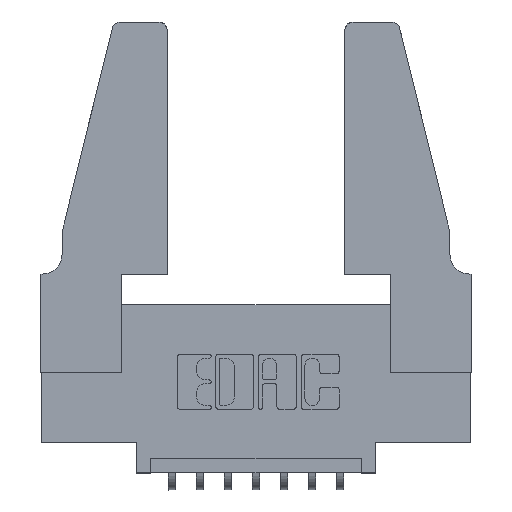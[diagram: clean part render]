
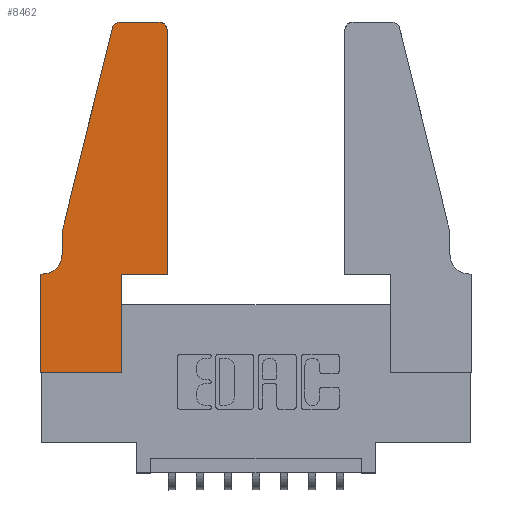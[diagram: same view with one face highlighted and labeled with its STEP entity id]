
A CAD part, top view. The second image highlights one B-rep face of the part: STEP entity #8462.
In plain terms, the highlighted planar face has unit normal (0, 0, 1).
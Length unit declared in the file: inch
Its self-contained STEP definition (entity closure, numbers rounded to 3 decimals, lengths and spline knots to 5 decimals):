
#113 = ORIENTED_EDGE ( 'NONE', *, *, #2184, .T. ) ;
#610 = VERTEX_POINT ( 'NONE', #11148 ) ;
#645 = DIRECTION ( 'NONE',  ( 0., 0., 1. ) ) ;
#992 = DIRECTION ( 'NONE',  ( -0.239, -0.971, 0. ) ) ;
#1128 = VERTEX_POINT ( 'NONE', #3103 ) ;
#1133 = CARTESIAN_POINT ( 'NONE',  ( 0.25487, 1.22718, 0.37 ) ) ;
#1304 = VECTOR ( 'NONE', #4880, 39.37008 ) ;
#1329 = EDGE_CURVE ( 'NONE', #610, #11386, #11660, .T. ) ;
#1362 = VERTEX_POINT ( 'NONE', #4406 ) ;
#1475 = CARTESIAN_POINT ( 'NONE',  ( 0.4505, 0.35, 0.37 ) ) ;
#1483 = VECTOR ( 'NONE', #10228, 39.37008 ) ;
#1531 = DIRECTION ( 'NONE',  ( 1., 0., 0. ) ) ;
#1594 = CARTESIAN_POINT ( 'NONE',  ( 0.0755, 0.5, 0.37 ) ) ;
#1610 = LINE ( 'NONE', #6700, #1304 ) ;
#2184 = EDGE_CURVE ( 'NONE', #7097, #1362, #9536, .T. ) ;
#2194 = ORIENTED_EDGE ( 'NONE', *, *, #4125, .T. ) ;
#2201 = ORIENTED_EDGE ( 'NONE', *, *, #6416, .T. ) ;
#2238 = VECTOR ( 'NONE', #10749, 39.37008 ) ;
#2318 = CARTESIAN_POINT ( 'NONE',  ( 0.4505, 0.35, 0.37 ) ) ;
#2446 = ORIENTED_EDGE ( 'NONE', *, *, #8698, .T. ) ;
#2585 = CARTESIAN_POINT ( 'NONE',  ( 0., 0., 0.37 ) ) ;
#2782 = CARTESIAN_POINT ( 'NONE',  ( 0.4505, 1.22, 0.37 ) ) ;
#3103 = CARTESIAN_POINT ( 'NONE',  ( 0.2865, 0.35, 0.37 ) ) ;
#3108 = CARTESIAN_POINT ( 'NONE',  ( 0.0755, 0.5, 0.37 ) ) ;
#3362 = DIRECTION ( 'NONE',  ( 0., 0., 1. ) ) ;
#3425 = LINE ( 'NONE', #9202, #6232 ) ;
#3544 = AXIS2_PLACEMENT_3D ( 'NONE', #6188, #3362, #1531 ) ;
#3649 = DIRECTION ( 'NONE',  ( 0., 0., 1. ) ) ;
#3719 = LINE ( 'NONE', #6308, #1483 ) ;
#3904 = CARTESIAN_POINT ( 'NONE',  ( 0.0755, 0.5, 0.37 ) ) ;
#4098 = ORIENTED_EDGE ( 'NONE', *, *, #5721, .T. ) ;
#4102 = VERTEX_POINT ( 'NONE', #9892 ) ;
#4125 = EDGE_CURVE ( 'NONE', #1128, #4346, #9208, .T. ) ;
#4147 = DIRECTION ( 'NONE',  ( 0., -1., 0. ) ) ;
#4346 = VERTEX_POINT ( 'NONE', #2318 ) ;
#4406 = CARTESIAN_POINT ( 'NONE',  ( 0.284, 1.25, 0.37 ) ) ;
#4829 = AXIS2_PLACEMENT_3D ( 'NONE', #8560, #9566, #10630 ) ;
#4880 = DIRECTION ( 'NONE',  ( 0., 1., 0. ) ) ;
#4893 = DIRECTION ( 'NONE',  ( -1., 0., 0. ) ) ;
#5330 = EDGE_CURVE ( 'NONE', #4346, #10936, #10996, .T. ) ;
#5580 = CARTESIAN_POINT ( 'NONE',  ( 0.0755, 0.42, 0.37 ) ) ;
#5721 = EDGE_CURVE ( 'NONE', #4102, #1128, #1610, .T. ) ;
#5824 = ORIENTED_EDGE ( 'NONE', *, *, #10765, .T. ) ;
#5925 = ORIENTED_EDGE ( 'NONE', *, *, #1329, .T. ) ;
#6145 = EDGE_CURVE ( 'NONE', #9162, #12372, #9012, .T. ) ;
#6188 = CARTESIAN_POINT ( 'NONE',  ( 0.4205, 1.22, 0.37 ) ) ;
#6232 = VECTOR ( 'NONE', #12234, 39.37008 ) ;
#6308 = CARTESIAN_POINT ( 'NONE',  ( 0., 0., 0.37 ) ) ;
#6384 = DIRECTION ( 'NONE',  ( 1., 0., 0. ) ) ;
#6416 = EDGE_CURVE ( 'NONE', #10936, #7097, #6638, .T. ) ;
#6452 = ORIENTED_EDGE ( 'NONE', *, *, #10562, .T. ) ;
#6454 = EDGE_CURVE ( 'NONE', #1362, #9162, #8845, .T. ) ;
#6638 = CIRCLE ( 'NONE', #3544, 0.03 ) ;
#6700 = CARTESIAN_POINT ( 'NONE',  ( 0.2865, 0.35, 0.37 ) ) ;
#7031 = CIRCLE ( 'NONE', #4829, 0.07 ) ;
#7097 = VERTEX_POINT ( 'NONE', #11101 ) ;
#7924 = ORIENTED_EDGE ( 'NONE', *, *, #11823, .T. ) ;
#8255 = PLANE ( 'NONE',  #9185 ) ;
#8291 = CARTESIAN_POINT ( 'NONE',  ( 0., 0.35, 0.37 ) ) ;
#8446 = CARTESIAN_POINT ( 'NONE',  ( 0.2605, 1.25, 0.37 ) ) ;
#8462 = ADVANCED_FACE ( 'NONE', ( #9123 ), #8255, .T. ) ;
#8465 = VECTOR ( 'NONE', #4147, 39.37008 ) ;
#8491 = VERTEX_POINT ( 'NONE', #2585 ) ;
#8505 = VECTOR ( 'NONE', #9828, 39.37008 ) ;
#8554 = ORIENTED_EDGE ( 'NONE', *, *, #6145, .T. ) ;
#8560 = CARTESIAN_POINT ( 'NONE',  ( 0.0055, 0.42, 0.37 ) ) ;
#8604 = VERTEX_POINT ( 'NONE', #5580 ) ;
#8698 = EDGE_CURVE ( 'NONE', #8604, #610, #7031, .T. ) ;
#8845 = CIRCLE ( 'NONE', #9014, 0.03 ) ;
#8893 = CARTESIAN_POINT ( 'NONE',  ( 0.0755, 0.35, 0.37 ) ) ;
#8925 = VECTOR ( 'NONE', #4893, 39.37008 ) ;
#9012 = LINE ( 'NONE', #3904, #12324 ) ;
#9014 = AXIS2_PLACEMENT_3D ( 'NONE', #12148, #3649, #11237 ) ;
#9123 = FACE_OUTER_BOUND ( 'NONE', #10285, .T. ) ;
#9162 = VERTEX_POINT ( 'NONE', #1133 ) ;
#9185 = AXIS2_PLACEMENT_3D ( 'NONE', #8291, #645, #6384 ) ;
#9202 = CARTESIAN_POINT ( 'NONE',  ( 0., 0., 0.37 ) ) ;
#9208 = LINE ( 'NONE', #9769, #2238 ) ;
#9329 = ORIENTED_EDGE ( 'NONE', *, *, #6454, .T. ) ;
#9388 = CARTESIAN_POINT ( 'NONE',  ( 0., 0.35, 0.37 ) ) ;
#9536 = LINE ( 'NONE', #8446, #8925 ) ;
#9566 = DIRECTION ( 'NONE',  ( 0., 0., -1. ) ) ;
#9769 = CARTESIAN_POINT ( 'NONE',  ( 0.4505, 0.35, 0.37 ) ) ;
#9828 = DIRECTION ( 'NONE',  ( -1., 0., 0. ) ) ;
#9892 = CARTESIAN_POINT ( 'NONE',  ( 0.2865, 0., 0.37 ) ) ;
#10143 = LINE ( 'NONE', #3108, #8465 ) ;
#10228 = DIRECTION ( 'NONE',  ( 1., 0., 0. ) ) ;
#10285 = EDGE_LOOP ( 'NONE', ( #113, #9329, #8554, #6452, #2446, #5925, #7924, #5824, #4098, #2194, #11251, #2201 ) ) ;
#10562 = EDGE_CURVE ( 'NONE', #12372, #8604, #10143, .T. ) ;
#10630 = DIRECTION ( 'NONE',  ( -1., 0., 0. ) ) ;
#10749 = DIRECTION ( 'NONE',  ( 1., 0., 0. ) ) ;
#10765 = EDGE_CURVE ( 'NONE', #8491, #4102, #3719, .T. ) ;
#10936 = VERTEX_POINT ( 'NONE', #2782 ) ;
#10996 = LINE ( 'NONE', #1475, #12333 ) ;
#11017 = DIRECTION ( 'NONE',  ( 0., 1., 0. ) ) ;
#11101 = CARTESIAN_POINT ( 'NONE',  ( 0.4205, 1.25, 0.37 ) ) ;
#11148 = CARTESIAN_POINT ( 'NONE',  ( 0.0055, 0.35, 0.37 ) ) ;
#11237 = DIRECTION ( 'NONE',  ( 1., 0., 0. ) ) ;
#11251 = ORIENTED_EDGE ( 'NONE', *, *, #5330, .T. ) ;
#11386 = VERTEX_POINT ( 'NONE', #9388 ) ;
#11660 = LINE ( 'NONE', #8893, #8505 ) ;
#11823 = EDGE_CURVE ( 'NONE', #11386, #8491, #3425, .T. ) ;
#12148 = CARTESIAN_POINT ( 'NONE',  ( 0.284, 1.22, 0.37 ) ) ;
#12234 = DIRECTION ( 'NONE',  ( 0., -1., 0. ) ) ;
#12324 = VECTOR ( 'NONE', #992, 39.37008 ) ;
#12333 = VECTOR ( 'NONE', #11017, 39.37008 ) ;
#12372 = VERTEX_POINT ( 'NONE', #1594 ) ;
